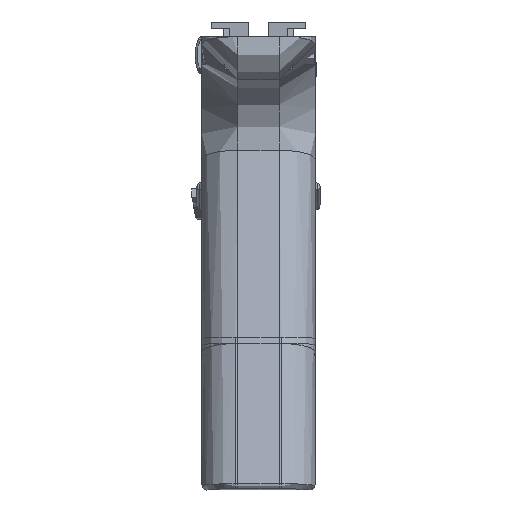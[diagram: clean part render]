
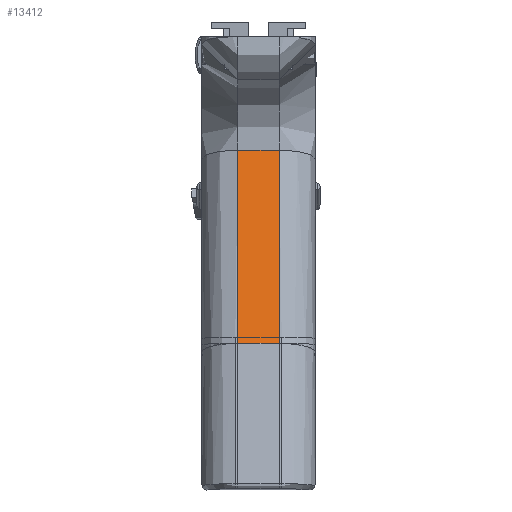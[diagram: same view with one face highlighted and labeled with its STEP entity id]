
A CAD part, front view. The second image highlights one B-rep face of the part: STEP entity #13412.
In plain terms, the highlighted face is planar.
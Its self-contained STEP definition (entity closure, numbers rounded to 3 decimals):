
#1048=PLANE('',#14635);
#1674=FACE_OUTER_BOUND('',#2452,.T.);
#2452=EDGE_LOOP('',(#11633,#11634,#11635,#11636));
#3480=LINE('',#23720,#4677);
#3636=LINE('',#24572,#4833);
#3637=LINE('',#24575,#4834);
#3638=LINE('',#24576,#4835);
#4677=VECTOR('',#17307,10.);
#4833=VECTOR('',#17711,10.);
#4834=VECTOR('',#17714,10.);
#4835=VECTOR('',#17715,10.);
#6297=VERTEX_POINT('',#23716);
#6298=VERTEX_POINT('',#23718);
#6437=VERTEX_POINT('',#24550);
#6440=VERTEX_POINT('',#24574);
#8024=EDGE_CURVE('',#6297,#6298,#3480,.T.);
#8250=EDGE_CURVE('',#6297,#6437,#3636,.T.);
#8251=EDGE_CURVE('',#6440,#6298,#3637,.T.);
#8252=EDGE_CURVE('',#6437,#6440,#3638,.T.);
#11633=ORIENTED_EDGE('',*,*,#8251,.F.);
#11634=ORIENTED_EDGE('',*,*,#8252,.F.);
#11635=ORIENTED_EDGE('',*,*,#8250,.F.);
#11636=ORIENTED_EDGE('',*,*,#8024,.T.);
#13412=ADVANCED_FACE('',(#1674),#1048,.T.);
#14635=AXIS2_PLACEMENT_3D('',#24573,#17712,#17713);
#17307=DIRECTION('',(0.,-0.249,0.969));
#17711=DIRECTION('',(-1.,0.,0.));
#17712=DIRECTION('center_axis',(0.,-0.969,
-0.249));
#17713=DIRECTION('ref_axis',(0.,-0.249,0.969));
#17714=DIRECTION('',(1.,0.,0.));
#17715=DIRECTION('',(0.,-0.249,0.969));
#23716=CARTESIAN_POINT('',(13.45,-71.634,19.877));
#23718=CARTESIAN_POINT('',(13.45,-83.628,66.536));
#23720=CARTESIAN_POINT('',(13.45,-83.554,66.245));
#24550=CARTESIAN_POINT('',(3.45,-71.634,19.877));
#24572=CARTESIAN_POINT('',(22.175,-71.634,19.877));
#24573=CARTESIAN_POINT('Origin',(22.175,-71.634,19.877));
#24574=CARTESIAN_POINT('',(3.45,-83.628,66.536));
#24575=CARTESIAN_POINT('',(22.175,-83.628,66.536));
#24576=CARTESIAN_POINT('',(3.45,-83.554,66.245));
